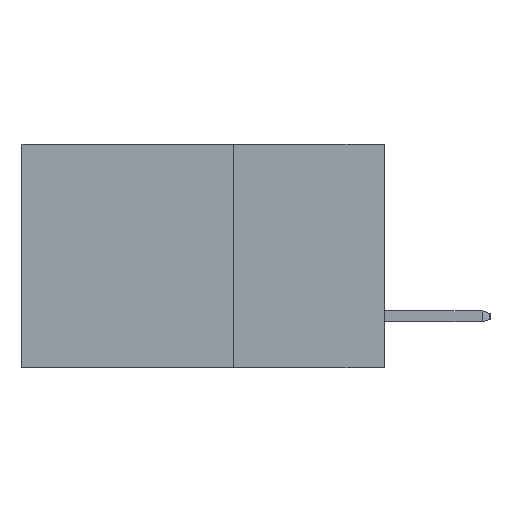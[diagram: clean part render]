
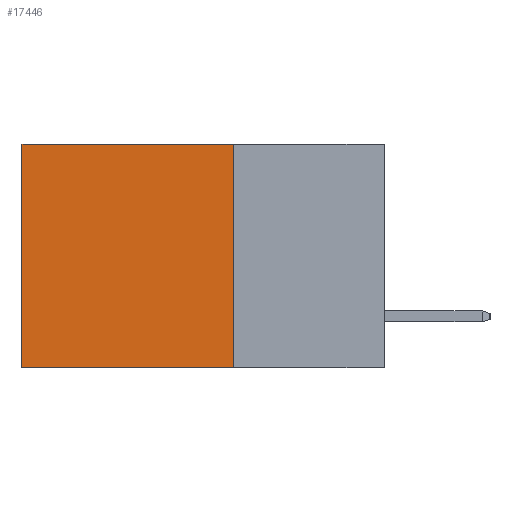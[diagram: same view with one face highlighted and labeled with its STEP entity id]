
A CAD part, left-side view. The second image highlights one B-rep face of the part: STEP entity #17446.
In plain terms, the highlighted planar face has unit normal (-1, 0, 0).
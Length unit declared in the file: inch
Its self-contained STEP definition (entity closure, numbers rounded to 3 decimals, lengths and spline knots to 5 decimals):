
#1355 = VERTEX_POINT ( 'NONE', #12204 ) ;
#3442 = PLANE ( 'NONE',  #14621 ) ;
#3539 = LINE ( 'NONE', #8689, #18628 ) ;
#4055 = DIRECTION ( 'NONE',  ( 0., 1., 0. ) ) ;
#4386 = EDGE_CURVE ( 'NONE', #7498, #1355, #14216, .T. ) ;
#4522 = EDGE_CURVE ( 'NONE', #15729, #1355, #3539, .T. ) ;
#4915 = DIRECTION ( 'NONE',  ( 1., 0., 0. ) ) ;
#6314 = ORIENTED_EDGE ( 'NONE', *, *, #4386, .T. ) ;
#6385 = VECTOR ( 'NONE', #10709, 39.37008 ) ;
#6829 = DIRECTION ( 'NONE',  ( 0., 1., 0. ) ) ;
#7242 = LINE ( 'NONE', #8253, #18390 ) ;
#7365 = FACE_OUTER_BOUND ( 'NONE', #16791, .T. ) ;
#7498 = VERTEX_POINT ( 'NONE', #14999 ) ;
#8253 = CARTESIAN_POINT ( 'NONE',  ( 0.298, 0.25, 0. ) ) ;
#8689 = CARTESIAN_POINT ( 'NONE',  ( 0.298, 0.25, -0.37 ) ) ;
#9060 = ORIENTED_EDGE ( 'NONE', *, *, #4522, .F. ) ;
#9077 = EDGE_CURVE ( 'NONE', #18168, #15729, #14267, .T. ) ;
#9773 = CARTESIAN_POINT ( 'NONE',  ( 0.298, 0.6, 0. ) ) ;
#10304 = VECTOR ( 'NONE', #16414, 39.37008 ) ;
#10709 = DIRECTION ( 'NONE',  ( 0., 0., -1. ) ) ;
#10847 = CARTESIAN_POINT ( 'NONE',  ( 0.298, 0.25, 0. ) ) ;
#11060 = ORIENTED_EDGE ( 'NONE', *, *, #9077, .F. ) ;
#11110 = CARTESIAN_POINT ( 'NONE',  ( 0.298, 0.25, 0. ) ) ;
#12138 = EDGE_CURVE ( 'NONE', #18168, #7498, #7242, .T. ) ;
#12204 = CARTESIAN_POINT ( 'NONE',  ( 0.298, 0.6, -0.37 ) ) ;
#13820 = CARTESIAN_POINT ( 'NONE',  ( 0.298, 0.25, 0. ) ) ;
#14216 = LINE ( 'NONE', #9773, #10304 ) ;
#14267 = LINE ( 'NONE', #10847, #6385 ) ;
#14621 = AXIS2_PLACEMENT_3D ( 'NONE', #13820, #4915, #15241 ) ;
#14999 = CARTESIAN_POINT ( 'NONE',  ( 0.298, 0.6, 0. ) ) ;
#15241 = DIRECTION ( 'NONE',  ( 0., 0., -1. ) ) ;
#15729 = VERTEX_POINT ( 'NONE', #16111 ) ;
#16111 = CARTESIAN_POINT ( 'NONE',  ( 0.298, 0.25, -0.37 ) ) ;
#16277 = ORIENTED_EDGE ( 'NONE', *, *, #12138, .T. ) ;
#16414 = DIRECTION ( 'NONE',  ( 0., 0., -1. ) ) ;
#16791 = EDGE_LOOP ( 'NONE', ( #6314, #9060, #11060, #16277 ) ) ;
#17446 = ADVANCED_FACE ( 'NONE', ( #7365 ), #3442, .F. ) ;
#18168 = VERTEX_POINT ( 'NONE', #11110 ) ;
#18390 = VECTOR ( 'NONE', #6829, 39.37008 ) ;
#18628 = VECTOR ( 'NONE', #4055, 39.37008 ) ;
